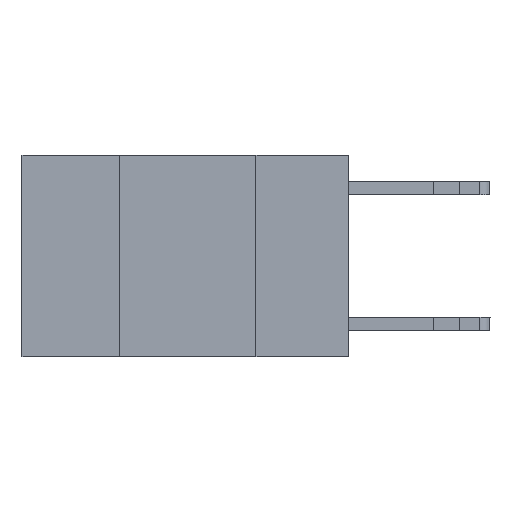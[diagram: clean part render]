
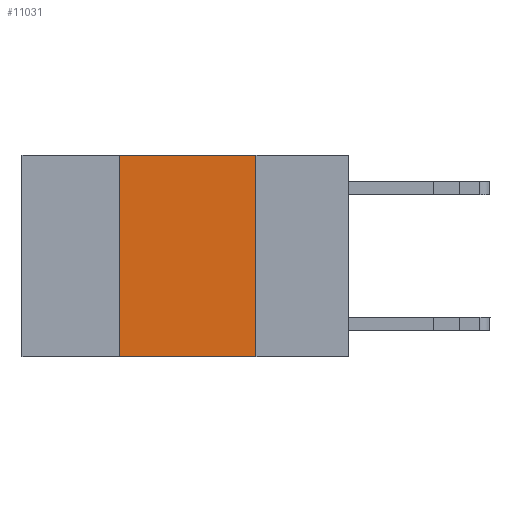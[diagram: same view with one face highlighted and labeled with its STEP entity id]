
A CAD part, left-side view. The second image highlights one B-rep face of the part: STEP entity #11031.
In plain terms, the highlighted planar face has unit normal (-1, 0, 0).
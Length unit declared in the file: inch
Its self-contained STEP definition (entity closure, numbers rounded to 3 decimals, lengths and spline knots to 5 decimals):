
#241 = ORIENTED_EDGE ( 'NONE', *, *, #4563, .F. ) ;
#983 = ORIENTED_EDGE ( 'NONE', *, *, #15779, .F. ) ;
#1421 = CARTESIAN_POINT ( 'NONE',  ( 0., 0.42, 0. ) ) ;
#1471 = EDGE_LOOP ( 'NONE', ( #241, #983, #2501, #2908 ) ) ;
#1594 = VERTEX_POINT ( 'NONE', #6369 ) ;
#1696 = VECTOR ( 'NONE', #14003, 39.37008 ) ;
#2501 = ORIENTED_EDGE ( 'NONE', *, *, #13370, .F. ) ;
#2760 = AXIS2_PLACEMENT_3D ( 'NONE', #18065, #8678, #19651 ) ;
#2908 = ORIENTED_EDGE ( 'NONE', *, *, #8104, .T. ) ;
#2911 = VECTOR ( 'NONE', #6107, 39.37008 ) ;
#2916 = DIRECTION ( 'NONE',  ( 0., -1., 0. ) ) ;
#2943 = CARTESIAN_POINT ( 'NONE',  ( 0., 0.17, 0. ) ) ;
#3900 = CARTESIAN_POINT ( 'NONE',  ( 0., 0.17, -0.37 ) ) ;
#4563 = EDGE_CURVE ( 'NONE', #16386, #9035, #11778, .T. ) ;
#5902 = LINE ( 'NONE', #1421, #1696 ) ;
#6107 = DIRECTION ( 'NONE',  ( 0., 0., -1. ) ) ;
#6369 = CARTESIAN_POINT ( 'NONE',  ( 0., 0.42, -0.37 ) ) ;
#6842 = DIRECTION ( 'NONE',  ( 0., -1., 0. ) ) ;
#6984 = VECTOR ( 'NONE', #6842, 39.37008 ) ;
#8104 = EDGE_CURVE ( 'NONE', #1594, #9035, #11664, .T. ) ;
#8678 = DIRECTION ( 'NONE',  ( 1., 0., 0. ) ) ;
#9035 = VERTEX_POINT ( 'NONE', #3900 ) ;
#11031 = ADVANCED_FACE ( 'NONE', ( #13033 ), #11794, .F. ) ;
#11664 = LINE ( 'NONE', #17789, #6984 ) ;
#11778 = LINE ( 'NONE', #2943, #2911 ) ;
#11794 = PLANE ( 'NONE',  #2760 ) ;
#12103 = CARTESIAN_POINT ( 'NONE',  ( 0., 0.17, 0. ) ) ;
#13033 = FACE_OUTER_BOUND ( 'NONE', #1471, .T. ) ;
#13107 = VERTEX_POINT ( 'NONE', #19432 ) ;
#13370 = EDGE_CURVE ( 'NONE', #1594, #13107, #5902, .T. ) ;
#13876 = LINE ( 'NONE', #13882, #17077 ) ;
#13882 = CARTESIAN_POINT ( 'NONE',  ( 0., 0.6, 0. ) ) ;
#14003 = DIRECTION ( 'NONE',  ( 0., 0., 1. ) ) ;
#15779 = EDGE_CURVE ( 'NONE', #13107, #16386, #13876, .T. ) ;
#16386 = VERTEX_POINT ( 'NONE', #12103 ) ;
#17077 = VECTOR ( 'NONE', #2916, 39.37008 ) ;
#17789 = CARTESIAN_POINT ( 'NONE',  ( 0., 0.6, -0.37 ) ) ;
#18065 = CARTESIAN_POINT ( 'NONE',  ( 0., 0.6, 0. ) ) ;
#19432 = CARTESIAN_POINT ( 'NONE',  ( 0., 0.42, 0. ) ) ;
#19651 = DIRECTION ( 'NONE',  ( 0., 0., -1. ) ) ;
